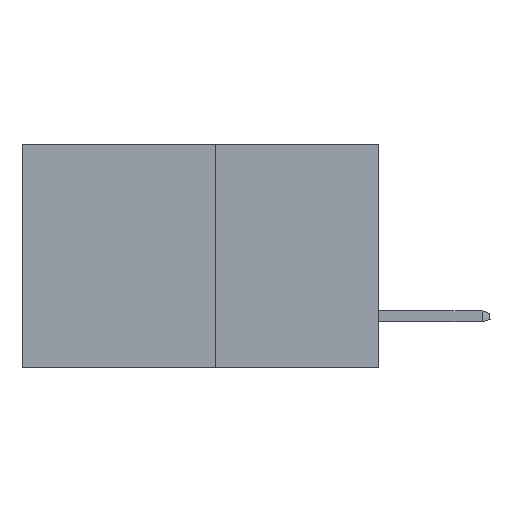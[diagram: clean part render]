
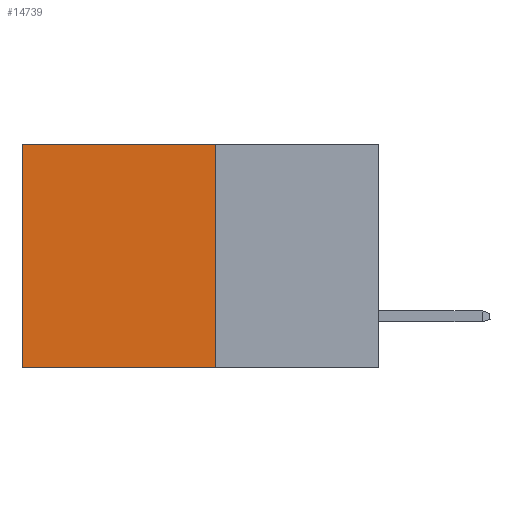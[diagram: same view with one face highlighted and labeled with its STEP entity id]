
A CAD part, left-side view. The second image highlights one B-rep face of the part: STEP entity #14739.
In plain terms, the highlighted planar face has unit normal (-1, 0, 0).
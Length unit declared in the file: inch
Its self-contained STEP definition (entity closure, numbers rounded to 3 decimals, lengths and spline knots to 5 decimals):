
#1151 = CARTESIAN_POINT ( 'NONE',  ( 0.277, 0.27, 0. ) ) ;
#2303 = LINE ( 'NONE', #7484, #14360 ) ;
#4047 = CARTESIAN_POINT ( 'NONE',  ( 0.277, 0.59, 0. ) ) ;
#4254 = CARTESIAN_POINT ( 'NONE',  ( 0.277, 0.27, 0. ) ) ;
#6064 = LINE ( 'NONE', #9490, #18085 ) ;
#6096 = CARTESIAN_POINT ( 'NONE',  ( 0.277, 0.27, -0.37 ) ) ;
#6332 = ORIENTED_EDGE ( 'NONE', *, *, #15949, .F. ) ;
#6673 = DIRECTION ( 'NONE',  ( 0., 1., 0. ) ) ;
#7083 = ORIENTED_EDGE ( 'NONE', *, *, #7360, .F. ) ;
#7360 = EDGE_CURVE ( 'NONE', #9007, #8292, #6064, .T. ) ;
#7484 = CARTESIAN_POINT ( 'NONE',  ( 0.277, 0.59, -0.37 ) ) ;
#7486 = LINE ( 'NONE', #20377, #19500 ) ;
#8292 = VERTEX_POINT ( 'NONE', #14883 ) ;
#9007 = VERTEX_POINT ( 'NONE', #6096 ) ;
#9354 = VECTOR ( 'NONE', #6673, 39.37008 ) ;
#9490 = CARTESIAN_POINT ( 'NONE',  ( 0.277, 0.27, -0.37 ) ) ;
#9596 = DIRECTION ( 'NONE',  ( 0., 1., 0. ) ) ;
#10119 = EDGE_LOOP ( 'NONE', ( #26681, #7083, #6332, #27798 ) ) ;
#10720 = DIRECTION ( 'NONE',  ( 0., 0., -1. ) ) ;
#11308 = DIRECTION ( 'NONE',  ( 1., 0., 0. ) ) ;
#14360 = VECTOR ( 'NONE', #24233, 39.37008 ) ;
#14739 = ADVANCED_FACE ( 'NONE', ( #23999 ), #18474, .F. ) ;
#14883 = CARTESIAN_POINT ( 'NONE',  ( 0.277, 0.59, -0.37 ) ) ;
#15949 = EDGE_CURVE ( 'NONE', #22077, #9007, #7486, .T. ) ;
#16059 = CARTESIAN_POINT ( 'NONE',  ( 0.277, 0.27, -0.37 ) ) ;
#16419 = AXIS2_PLACEMENT_3D ( 'NONE', #16059, #11308, #28028 ) ;
#18085 = VECTOR ( 'NONE', #9596, 39.37008 ) ;
#18474 = PLANE ( 'NONE',  #16419 ) ;
#19491 = EDGE_CURVE ( 'NONE', #22077, #22189, #22120, .T. ) ;
#19500 = VECTOR ( 'NONE', #10720, 39.37008 ) ;
#20377 = CARTESIAN_POINT ( 'NONE',  ( 0.277, 0.27, -0.37 ) ) ;
#22077 = VERTEX_POINT ( 'NONE', #1151 ) ;
#22120 = LINE ( 'NONE', #4254, #9354 ) ;
#22189 = VERTEX_POINT ( 'NONE', #4047 ) ;
#22492 = EDGE_CURVE ( 'NONE', #22189, #8292, #2303, .T. ) ;
#23999 = FACE_OUTER_BOUND ( 'NONE', #10119, .T. ) ;
#24233 = DIRECTION ( 'NONE',  ( 0., 0., -1. ) ) ;
#26681 = ORIENTED_EDGE ( 'NONE', *, *, #22492, .T. ) ;
#27798 = ORIENTED_EDGE ( 'NONE', *, *, #19491, .T. ) ;
#28028 = DIRECTION ( 'NONE',  ( 0., 0., -1. ) ) ;
